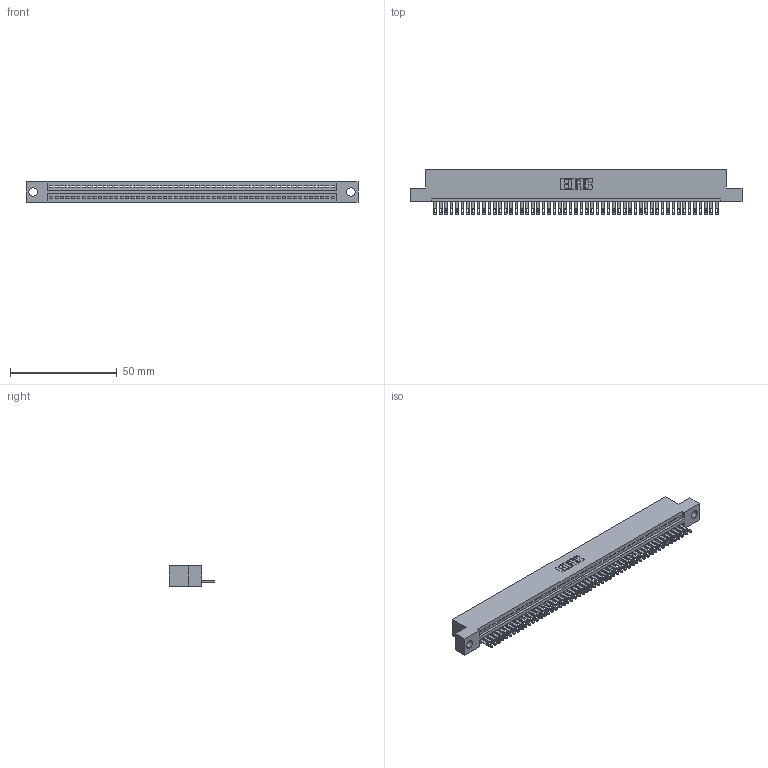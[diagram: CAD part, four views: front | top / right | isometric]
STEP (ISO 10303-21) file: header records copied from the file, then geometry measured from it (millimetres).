
FILE_DESCRIPTION (( 'STEP AP203' ), '1' );
FILE_NAME ('345-053-500-104.STEP', '2021-05-28T15:28:05', ( '' ), ( '' ), 'SwSTEP 2.0', 'SolidWorks 2020', '' );
FILE_SCHEMA (( 'CONFIG_CONTROL_DESIGN' ));
Length unit declared in the file: inch
Products named in the file (3): 345-292-001_345-293-100; 345-053-500-104; 345 Part_Flush Mounting Lugs - 0.156 Dia-TI
Assembly tree (54 placements, depth 2):
  345-053-500-104
    345 Part_Flush Mounting Lugs - 0.156 Dia-TI
    345-292-001_345-293-100  x53
Bounding box: 155.83 x 21.51 x 9.4 mm (x, y, z)
Volume: 14817.8 mm3; surface area: 19802.5 mm2
Topology: 54 solids, 54 shells, 3002 faces, 9281 edges, 6186 vertices
Faces by surface type: plane 1896, cylinder 1106
Entity records: 38757 total; most frequent: CARTESIAN_POINT 6721, ORIENTED_EDGE 6706, DIRECTION 5855, EDGE_CURVE 3353, VECTOR 3005, LINE 3005, VERTEX_POINT 2234, AXIS2_PLACEMENT_3D 1425
